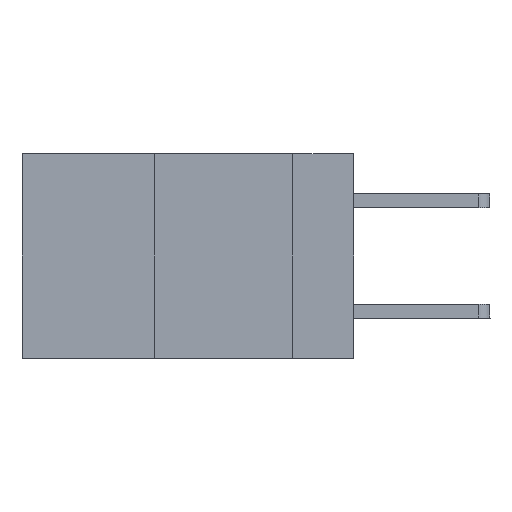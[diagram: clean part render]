
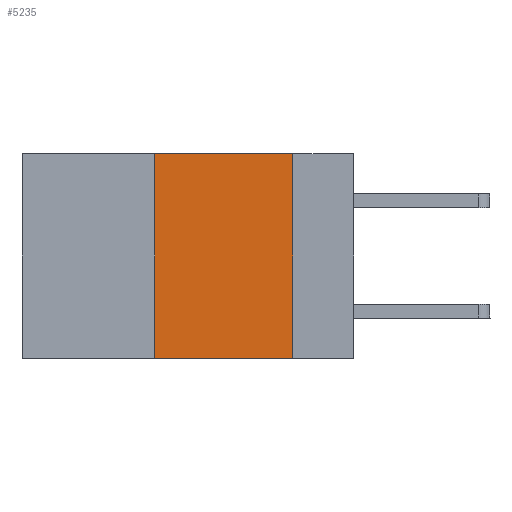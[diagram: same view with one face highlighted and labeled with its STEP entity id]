
A CAD part, left-side view. The second image highlights one B-rep face of the part: STEP entity #5235.
In plain terms, the highlighted planar face has unit normal (-1, 0, 0).
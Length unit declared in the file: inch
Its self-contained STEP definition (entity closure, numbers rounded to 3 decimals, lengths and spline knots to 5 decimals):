
#96 = ORIENTED_EDGE ( 'NONE', *, *, #4673, .F. ) ;
#124 = ORIENTED_EDGE ( 'NONE', *, *, #3220, .F. ) ;
#425 = VECTOR ( 'NONE', #3363, 39.37008 ) ;
#659 = CARTESIAN_POINT ( 'NONE',  ( 0., 0.36, 0. ) ) ;
#1241 = EDGE_CURVE ( 'NONE', #4960, #4077, #8768, .T. ) ;
#1975 = DIRECTION ( 'NONE',  ( 0., 0., -1. ) ) ;
#2289 = VECTOR ( 'NONE', #11469, 39.37008 ) ;
#2979 = DIRECTION ( 'NONE',  ( 0., -1., 0. ) ) ;
#3220 = EDGE_CURVE ( 'NONE', #4077, #5377, #13161, .T. ) ;
#3363 = DIRECTION ( 'NONE',  ( 0., 0., 1. ) ) ;
#4077 = VERTEX_POINT ( 'NONE', #659 ) ;
#4673 = EDGE_CURVE ( 'NONE', #5377, #8862, #13905, .T. ) ;
#4960 = VERTEX_POINT ( 'NONE', #10503 ) ;
#5235 = ADVANCED_FACE ( 'NONE', ( #8719 ), #5331, .F. ) ;
#5331 = PLANE ( 'NONE',  #13064 ) ;
#5377 = VERTEX_POINT ( 'NONE', #12140 ) ;
#5986 = VECTOR ( 'NONE', #2979, 39.37008 ) ;
#6135 = LINE ( 'NONE', #12603, #5986 ) ;
#6304 = EDGE_CURVE ( 'NONE', #4960, #8862, #6135, .T. ) ;
#7043 = EDGE_LOOP ( 'NONE', ( #96, #124, #11834, #7139 ) ) ;
#7139 = ORIENTED_EDGE ( 'NONE', *, *, #6304, .T. ) ;
#7608 = CARTESIAN_POINT ( 'NONE',  ( 0., 0.36, 0. ) ) ;
#8238 = VECTOR ( 'NONE', #13022, 39.37008 ) ;
#8577 = CARTESIAN_POINT ( 'NONE',  ( 0., 0.6, 0. ) ) ;
#8719 = FACE_OUTER_BOUND ( 'NONE', #7043, .T. ) ;
#8768 = LINE ( 'NONE', #7608, #425 ) ;
#8862 = VERTEX_POINT ( 'NONE', #13222 ) ;
#10503 = CARTESIAN_POINT ( 'NONE',  ( 0., 0.36, -0.37 ) ) ;
#11469 = DIRECTION ( 'NONE',  ( 0., 0., -1. ) ) ;
#11679 = CARTESIAN_POINT ( 'NONE',  ( 0., 0.11, 0. ) ) ;
#11733 = DIRECTION ( 'NONE',  ( 1., 0., 0. ) ) ;
#11834 = ORIENTED_EDGE ( 'NONE', *, *, #1241, .F. ) ;
#12140 = CARTESIAN_POINT ( 'NONE',  ( 0., 0.11, 0. ) ) ;
#12603 = CARTESIAN_POINT ( 'NONE',  ( 0., 0.6, -0.37 ) ) ;
#13022 = DIRECTION ( 'NONE',  ( 0., -1., 0. ) ) ;
#13064 = AXIS2_PLACEMENT_3D ( 'NONE', #8577, #11733, #1975 ) ;
#13161 = LINE ( 'NONE', #14187, #8238 ) ;
#13222 = CARTESIAN_POINT ( 'NONE',  ( 0., 0.11, -0.37 ) ) ;
#13905 = LINE ( 'NONE', #11679, #2289 ) ;
#14187 = CARTESIAN_POINT ( 'NONE',  ( 0., 0.6, 0. ) ) ;
